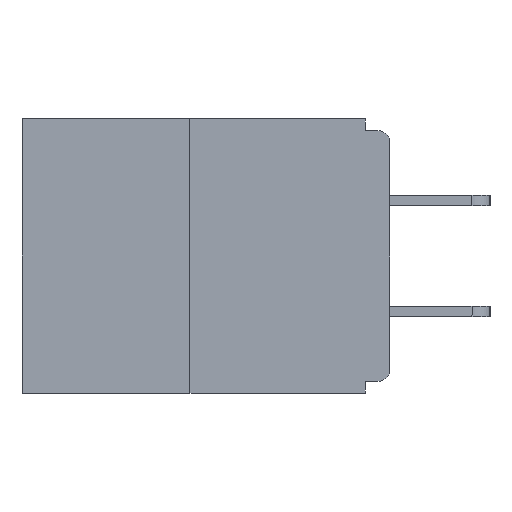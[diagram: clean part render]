
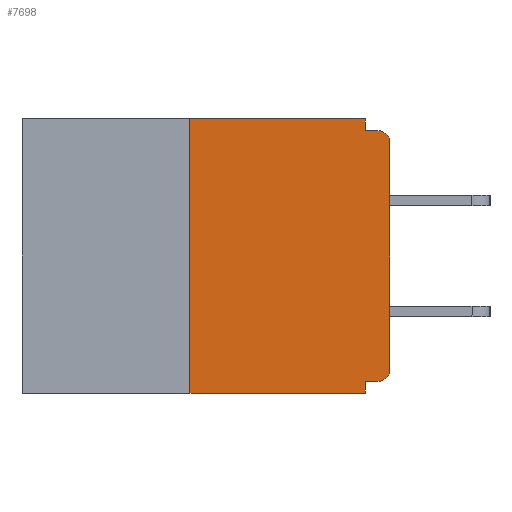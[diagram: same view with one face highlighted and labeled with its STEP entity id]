
A CAD part, left-side view. The second image highlights one B-rep face of the part: STEP entity #7698.
In plain terms, the highlighted planar face has unit normal (-1, 0, 0).
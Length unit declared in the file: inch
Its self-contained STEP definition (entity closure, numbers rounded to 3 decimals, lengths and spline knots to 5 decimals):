
#85 = VERTEX_POINT ( 'NONE', #7370 ) ;
#101 = LINE ( 'NONE', #6556, #239 ) ;
#163 = VERTEX_POINT ( 'NONE', #10221 ) ;
#239 = VECTOR ( 'NONE', #4733, 39.37008 ) ;
#310 = DIRECTION ( 'NONE',  ( 0., 0., -1. ) ) ;
#359 = EDGE_CURVE ( 'NONE', #547, #11432, #9426, .T. ) ;
#370 = LINE ( 'NONE', #10640, #9317 ) ;
#398 = DIRECTION ( 'NONE',  ( 0., 0., 1. ) ) ;
#500 = DIRECTION ( 'NONE',  ( 0., 0., -1. ) ) ;
#547 = VERTEX_POINT ( 'NONE', #3517 ) ;
#767 = VERTEX_POINT ( 'NONE', #6569 ) ;
#849 = CARTESIAN_POINT ( 'NONE',  ( 0., 0.031, 0. ) ) ;
#981 = CARTESIAN_POINT ( 'NONE',  ( 0., 0.46, 0. ) ) ;
#1067 = DIRECTION ( 'NONE',  ( 0., 0., -1. ) ) ;
#1264 = AXIS2_PLACEMENT_3D ( 'NONE', #2341, #3326, #5177 ) ;
#1423 = PLANE ( 'NONE',  #1264 ) ;
#1469 = AXIS2_PLACEMENT_3D ( 'NONE', #11344, #3865, #1067 ) ;
#1588 = DIRECTION ( 'NONE',  ( 0., 0., 1. ) ) ;
#1684 = ORIENTED_EDGE ( 'NONE', *, *, #11139, .F. ) ;
#1728 = EDGE_CURVE ( 'NONE', #11807, #2909, #7828, .T. ) ;
#1972 = ORIENTED_EDGE ( 'NONE', *, *, #7571, .F. ) ;
#2070 = CARTESIAN_POINT ( 'NONE',  ( 0., 0.031, -0.343 ) ) ;
#2185 = DIRECTION ( 'NONE',  ( 0., 1., 0. ) ) ;
#2199 = ORIENTED_EDGE ( 'NONE', *, *, #4756, .T. ) ;
#2233 = DIRECTION ( 'NONE',  ( 0., 0., -1. ) ) ;
#2341 = CARTESIAN_POINT ( 'NONE',  ( 0., 0.46, 0. ) ) ;
#2372 = CARTESIAN_POINT ( 'NONE',  ( 0., 0.031, -0.328 ) ) ;
#2466 = CARTESIAN_POINT ( 'NONE',  ( 0., 0., -0.313 ) ) ;
#2471 = DIRECTION ( 'NONE',  ( 0., -1., 0. ) ) ;
#2519 = VERTEX_POINT ( 'NONE', #4099 ) ;
#2833 = VECTOR ( 'NONE', #6548, 39.37008 ) ;
#2909 = VERTEX_POINT ( 'NONE', #3964 ) ;
#2972 = ORIENTED_EDGE ( 'NONE', *, *, #359, .T. ) ;
#3019 = VERTEX_POINT ( 'NONE', #6830 ) ;
#3198 = CARTESIAN_POINT ( 'NONE',  ( 0., 0.015, -0.313 ) ) ;
#3326 = DIRECTION ( 'NONE',  ( 1., 0., 0. ) ) ;
#3517 = CARTESIAN_POINT ( 'NONE',  ( 0., 0.015, -0.328 ) ) ;
#3865 = DIRECTION ( 'NONE',  ( -1., 0., 0. ) ) ;
#3964 = CARTESIAN_POINT ( 'NONE',  ( 0., 0.031, -0.343 ) ) ;
#4099 = CARTESIAN_POINT ( 'NONE',  ( 0., 0.25, -0.343 ) ) ;
#4303 = EDGE_CURVE ( 'NONE', #163, #767, #101, .T. ) ;
#4733 = DIRECTION ( 'NONE',  ( 0., -1., 0. ) ) ;
#4756 = EDGE_CURVE ( 'NONE', #2519, #2909, #7880, .T. ) ;
#4858 = LINE ( 'NONE', #981, #2833 ) ;
#5177 = DIRECTION ( 'NONE',  ( 0., 0., -1. ) ) ;
#5434 = FACE_OUTER_BOUND ( 'NONE', #11109, .T. ) ;
#5515 = LINE ( 'NONE', #9359, #6833 ) ;
#5833 = AXIS2_PLACEMENT_3D ( 'NONE', #3198, #9729, #500 ) ;
#5846 = VECTOR ( 'NONE', #2471, 39.37008 ) ;
#5943 = LINE ( 'NONE', #7742, #8403 ) ;
#6159 = CARTESIAN_POINT ( 'NONE',  ( 0., 0., 0. ) ) ;
#6304 = CARTESIAN_POINT ( 'NONE',  ( 0., 0.46, -0.343 ) ) ;
#6548 = DIRECTION ( 'NONE',  ( 0., -1., 0. ) ) ;
#6556 = CARTESIAN_POINT ( 'NONE',  ( 0., 0., -0.015 ) ) ;
#6569 = CARTESIAN_POINT ( 'NONE',  ( 0., 0.015, -0.015 ) ) ;
#6726 = VECTOR ( 'NONE', #1588, 39.37008 ) ;
#6830 = CARTESIAN_POINT ( 'NONE',  ( 0., 0.25, 0. ) ) ;
#6833 = VECTOR ( 'NONE', #2233, 39.37008 ) ;
#7000 = EDGE_CURVE ( 'NONE', #85, #767, #8941, .T. ) ;
#7370 = CARTESIAN_POINT ( 'NONE',  ( 0., 0., -0.03 ) ) ;
#7571 = EDGE_CURVE ( 'NONE', #3019, #7864, #4858, .T. ) ;
#7698 = ADVANCED_FACE ( 'NONE', ( #5434 ), #1423, .F. ) ;
#7742 = CARTESIAN_POINT ( 'NONE',  ( 0., 0.25, 0. ) ) ;
#7828 = LINE ( 'NONE', #2070, #10981 ) ;
#7864 = VERTEX_POINT ( 'NONE', #849 ) ;
#7880 = LINE ( 'NONE', #6304, #5846 ) ;
#8344 = ORIENTED_EDGE ( 'NONE', *, *, #11166, .F. ) ;
#8374 = ORIENTED_EDGE ( 'NONE', *, *, #4303, .F. ) ;
#8403 = VECTOR ( 'NONE', #398, 39.37008 ) ;
#8410 = EDGE_CURVE ( 'NONE', #11432, #85, #9786, .T. ) ;
#8779 = ORIENTED_EDGE ( 'NONE', *, *, #8410, .T. ) ;
#8941 = CIRCLE ( 'NONE', #1469, 0.015 ) ;
#9100 = EDGE_CURVE ( 'NONE', #547, #11807, #370, .T. ) ;
#9317 = VECTOR ( 'NONE', #2185, 39.37008 ) ;
#9359 = CARTESIAN_POINT ( 'NONE',  ( 0., 0.031, 0. ) ) ;
#9426 = CIRCLE ( 'NONE', #5833, 0.015 ) ;
#9599 = ORIENTED_EDGE ( 'NONE', *, *, #7000, .T. ) ;
#9729 = DIRECTION ( 'NONE',  ( -1., 0., 0. ) ) ;
#9786 = LINE ( 'NONE', #6159, #6726 ) ;
#10182 = ORIENTED_EDGE ( 'NONE', *, *, #9100, .F. ) ;
#10221 = CARTESIAN_POINT ( 'NONE',  ( 0., 0.031, -0.015 ) ) ;
#10640 = CARTESIAN_POINT ( 'NONE',  ( 0., 0., -0.328 ) ) ;
#10981 = VECTOR ( 'NONE', #310, 39.37008 ) ;
#11109 = EDGE_LOOP ( 'NONE', ( #1972, #8344, #2199, #11514, #10182, #2972, #8779, #9599, #8374, #1684 ) ) ;
#11139 = EDGE_CURVE ( 'NONE', #7864, #163, #5515, .T. ) ;
#11166 = EDGE_CURVE ( 'NONE', #2519, #3019, #5943, .T. ) ;
#11344 = CARTESIAN_POINT ( 'NONE',  ( 0., 0.015, -0.03 ) ) ;
#11432 = VERTEX_POINT ( 'NONE', #2466 ) ;
#11514 = ORIENTED_EDGE ( 'NONE', *, *, #1728, .F. ) ;
#11807 = VERTEX_POINT ( 'NONE', #2372 ) ;
